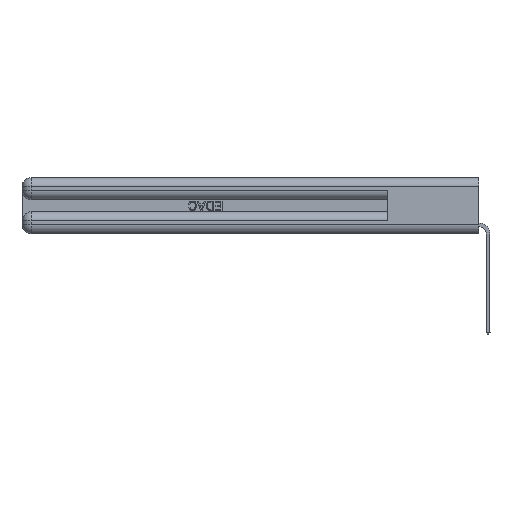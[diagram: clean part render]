
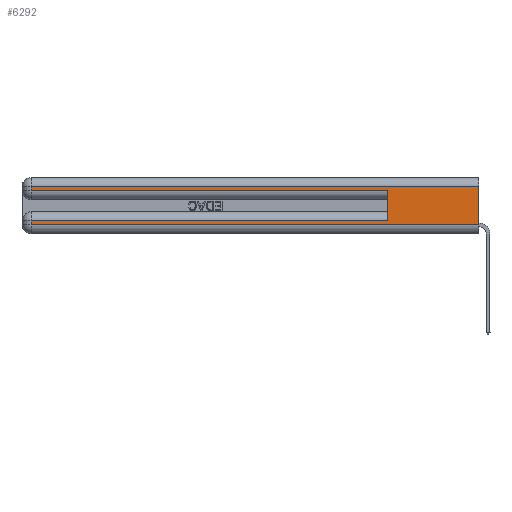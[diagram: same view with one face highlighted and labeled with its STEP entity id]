
A CAD part, left-side view. The second image highlights one B-rep face of the part: STEP entity #6292.
In plain terms, the highlighted planar face has unit normal (-1, 0, 0).
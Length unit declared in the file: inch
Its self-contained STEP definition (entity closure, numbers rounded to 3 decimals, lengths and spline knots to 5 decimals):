
#145 = LINE ( 'NONE', #28370, #5405 ) ;
#562 = EDGE_CURVE ( 'NONE', #28103, #19667, #27162, .T. ) ;
#1368 = CARTESIAN_POINT ( 'NONE',  ( 0., 2.94, 0.37 ) ) ;
#1981 = DIRECTION ( 'NONE',  ( 0., 1., 0. ) ) ;
#2102 = VERTEX_POINT ( 'NONE', #29267 ) ;
#2984 = VERTEX_POINT ( 'NONE', #4287 ) ;
#3228 = VECTOR ( 'NONE', #13188, 39.37008 ) ;
#3331 = DIRECTION ( 'NONE',  ( 0., 0., 1. ) ) ;
#3389 = LINE ( 'NONE', #17247, #12070 ) ;
#3742 = CARTESIAN_POINT ( 'NONE',  ( 0., 0.6, 0.085 ) ) ;
#3829 = DIRECTION ( 'NONE',  ( 0., 0., -1. ) ) ;
#4137 = ORIENTED_EDGE ( 'NONE', *, *, #4880, .F. ) ;
#4241 = CARTESIAN_POINT ( 'NONE',  ( 0., 0., 0.085 ) ) ;
#4287 = CARTESIAN_POINT ( 'NONE',  ( 0., 2.94, 0.06 ) ) ;
#4808 = PLANE ( 'NONE',  #7486 ) ;
#4880 = EDGE_CURVE ( 'NONE', #2102, #6546, #9461, .T. ) ;
#5228 = ORIENTED_EDGE ( 'NONE', *, *, #8437, .F. ) ;
#5267 = FACE_OUTER_BOUND ( 'NONE', #7320, .T. ) ;
#5405 = VECTOR ( 'NONE', #3331, 39.37008 ) ;
#6292 = ADVANCED_FACE ( 'NONE', ( #5267 ), #4808, .F. ) ;
#6336 = ORIENTED_EDGE ( 'NONE', *, *, #562, .T. ) ;
#6546 = VERTEX_POINT ( 'NONE', #29794 ) ;
#7320 = EDGE_LOOP ( 'NONE', ( #4137, #24061, #21510, #9746, #5228, #6336, #17233, #18428 ) ) ;
#7486 = AXIS2_PLACEMENT_3D ( 'NONE', #16710, #23656, #25610 ) ;
#7493 = DIRECTION ( 'NONE',  ( 0., 1., 0. ) ) ;
#7649 = LINE ( 'NONE', #16987, #24421 ) ;
#8437 = EDGE_CURVE ( 'NONE', #28103, #29235, #145, .T. ) ;
#8651 = VECTOR ( 'NONE', #28127, 39.37008 ) ;
#9461 = LINE ( 'NONE', #11730, #25744 ) ;
#9531 = VECTOR ( 'NONE', #19324, 39.37008 ) ;
#9615 = DIRECTION ( 'NONE',  ( 0., 0., -1. ) ) ;
#9720 = CARTESIAN_POINT ( 'NONE',  ( 0., 0., 0.285 ) ) ;
#9746 = ORIENTED_EDGE ( 'NONE', *, *, #19200, .T. ) ;
#11730 = CARTESIAN_POINT ( 'NONE',  ( 0., 0., 0.37 ) ) ;
#12070 = VECTOR ( 'NONE', #3829, 39.37008 ) ;
#12708 = CARTESIAN_POINT ( 'NONE',  ( 0., 2.94, 0.285 ) ) ;
#13188 = DIRECTION ( 'NONE',  ( 0., -1., 0. ) ) ;
#14042 = EDGE_CURVE ( 'NONE', #2984, #6546, #29176, .T. ) ;
#15432 = CARTESIAN_POINT ( 'NONE',  ( 0., 2.94, 0.31 ) ) ;
#16174 = VECTOR ( 'NONE', #1981, 39.37008 ) ;
#16312 = LINE ( 'NONE', #1368, #9531 ) ;
#16710 = CARTESIAN_POINT ( 'NONE',  ( 0., 0., 0.37 ) ) ;
#16987 = CARTESIAN_POINT ( 'NONE',  ( 0., 0., 0.31 ) ) ;
#17233 = ORIENTED_EDGE ( 'NONE', *, *, #19293, .T. ) ;
#17247 = CARTESIAN_POINT ( 'NONE',  ( 0., 2.94, 0.37 ) ) ;
#18428 = ORIENTED_EDGE ( 'NONE', *, *, #14042, .T. ) ;
#19200 = EDGE_CURVE ( 'NONE', #19323, #29235, #21185, .T. ) ;
#19293 = EDGE_CURVE ( 'NONE', #19667, #2984, #3389, .T. ) ;
#19323 = VERTEX_POINT ( 'NONE', #12708 ) ;
#19324 = DIRECTION ( 'NONE',  ( 0., 0., -1. ) ) ;
#19667 = VERTEX_POINT ( 'NONE', #22035 ) ;
#20992 = CARTESIAN_POINT ( 'NONE',  ( 0., 0.6, 0.285 ) ) ;
#21185 = LINE ( 'NONE', #9720, #8651 ) ;
#21510 = ORIENTED_EDGE ( 'NONE', *, *, #26123, .T. ) ;
#22035 = CARTESIAN_POINT ( 'NONE',  ( 0., 2.94, 0.085 ) ) ;
#22828 = CARTESIAN_POINT ( 'NONE',  ( 0., 0., 0.06 ) ) ;
#23656 = DIRECTION ( 'NONE',  ( 1., 0., 0. ) ) ;
#24061 = ORIENTED_EDGE ( 'NONE', *, *, #25375, .T. ) ;
#24421 = VECTOR ( 'NONE', #7493, 39.37008 ) ;
#25375 = EDGE_CURVE ( 'NONE', #2102, #25965, #7649, .T. ) ;
#25610 = DIRECTION ( 'NONE',  ( 0., 0., -1. ) ) ;
#25744 = VECTOR ( 'NONE', #9615, 39.37008 ) ;
#25965 = VERTEX_POINT ( 'NONE', #15432 ) ;
#26123 = EDGE_CURVE ( 'NONE', #25965, #19323, #16312, .T. ) ;
#27162 = LINE ( 'NONE', #4241, #16174 ) ;
#28103 = VERTEX_POINT ( 'NONE', #3742 ) ;
#28127 = DIRECTION ( 'NONE',  ( 0., -1., 0. ) ) ;
#28370 = CARTESIAN_POINT ( 'NONE',  ( 0., 0.6, 0.145 ) ) ;
#29176 = LINE ( 'NONE', #22828, #3228 ) ;
#29235 = VERTEX_POINT ( 'NONE', #20992 ) ;
#29267 = CARTESIAN_POINT ( 'NONE',  ( 0., 0., 0.31 ) ) ;
#29794 = CARTESIAN_POINT ( 'NONE',  ( 0., 0., 0.06 ) ) ;
